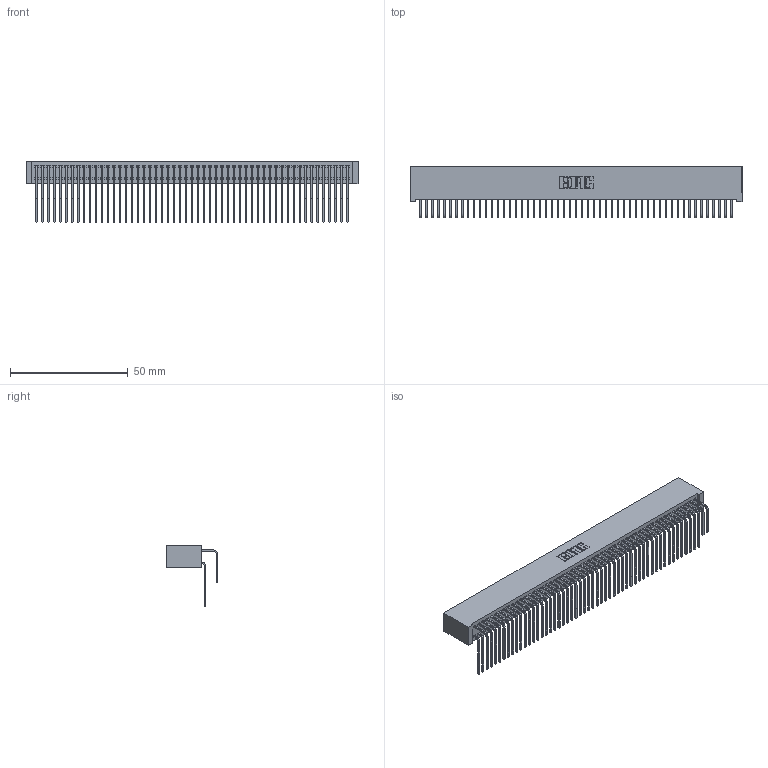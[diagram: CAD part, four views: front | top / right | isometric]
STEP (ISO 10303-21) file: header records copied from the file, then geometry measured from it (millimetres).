
FILE_DESCRIPTION (( 'STEP AP203' ), '1' );
FILE_NAME ('392-106-558-201.STEP', '2018-08-18T20:33:12', ( '' ), ( '' ), 'SwSTEP 2.0', 'SolidWorks 2016', '' );
FILE_SCHEMA (( 'CONFIG_CONTROL_DESIGN' ));
Length unit declared in the file: inch
Products named in the file (4): 345-292-001_558 Tail - 2; 392-106-558-201; 342 Part_Lugless; 345-292-001_558 559 Tail - 1
Assembly tree (107 placements, depth 2):
  392-106-558-201
    342 Part_Lugless
    345-292-001_558 559 Tail - 1  x53
    345-292-001_558 Tail - 2  x53
Bounding box: 140.87 x 21.91 x 25.78 mm (x, y, z)
Volume: 13760.1 mm3; surface area: 25881.4 mm2
Topology: 107 solids, 107 shells, 5826 faces, 17341 edges, 11418 vertices
Faces by surface type: plane 4090, cylinder 1736
Entity records: 34049 total; most frequent: CARTESIAN_POINT 5677, ORIENTED_EDGE 5562, DIRECTION 4805, EDGE_CURVE 2781, VECTOR 2621, LINE 2621, VERTEX_POINT 1850, AXIS2_PLACEMENT_3D 1092
